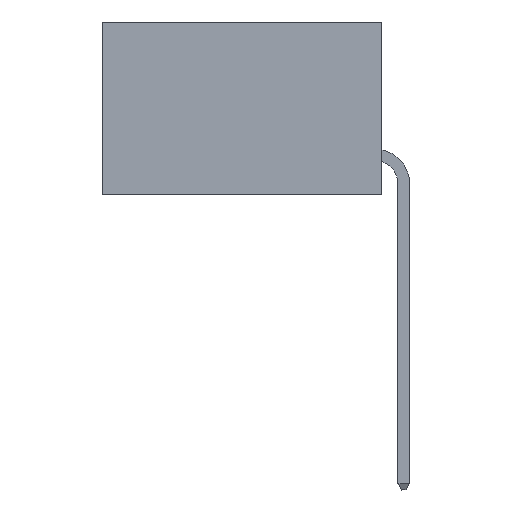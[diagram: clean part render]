
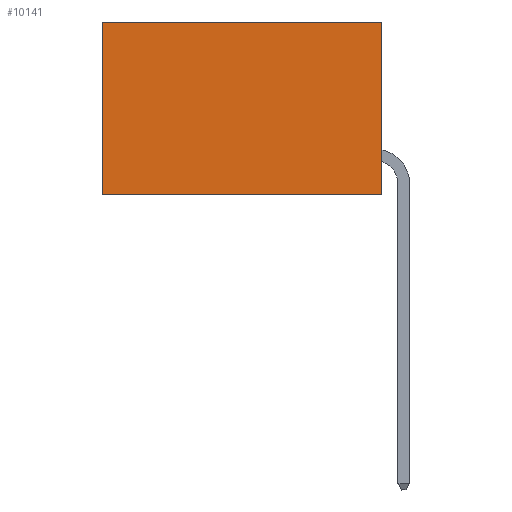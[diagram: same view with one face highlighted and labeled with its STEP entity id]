
A CAD part, left-side view. The second image highlights one B-rep face of the part: STEP entity #10141.
In plain terms, the highlighted planar face has unit normal (-1, 0, 0).
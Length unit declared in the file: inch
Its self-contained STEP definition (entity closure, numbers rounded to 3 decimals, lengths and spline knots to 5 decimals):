
#90 = VERTEX_POINT ( 'NONE', #14069 ) ;
#235 = CARTESIAN_POINT ( 'NONE',  ( 0.2875, 0., 0. ) ) ;
#974 = VERTEX_POINT ( 'NONE', #19655 ) ;
#2861 = VERTEX_POINT ( 'NONE', #24885 ) ;
#3293 = CARTESIAN_POINT ( 'NONE',  ( 0.2875, 0., -0.37 ) ) ;
#5614 = VECTOR ( 'NONE', #13836, 39.37008 ) ;
#5884 = EDGE_CURVE ( 'NONE', #14238, #2861, #18530, .T. ) ;
#6183 = PLANE ( 'NONE',  #18681 ) ;
#7469 = VECTOR ( 'NONE', #16303, 39.37008 ) ;
#7893 = VECTOR ( 'NONE', #18753, 39.37008 ) ;
#8208 = CARTESIAN_POINT ( 'NONE',  ( 0.2875, 0., 0. ) ) ;
#8600 = FACE_OUTER_BOUND ( 'NONE', #19274, .T. ) ;
#8960 = LINE ( 'NONE', #14454, #7469 ) ;
#10034 = ORIENTED_EDGE ( 'NONE', *, *, #5884, .T. ) ;
#10141 = ADVANCED_FACE ( 'NONE', ( #8600 ), #6183, .F. ) ;
#10660 = DIRECTION ( 'NONE',  ( 0., 0., -1. ) ) ;
#10783 = LINE ( 'NONE', #235, #5614 ) ;
#13058 = ORIENTED_EDGE ( 'NONE', *, *, #24590, .F. ) ;
#13836 = DIRECTION ( 'NONE',  ( 0., 0., -1. ) ) ;
#14012 = CARTESIAN_POINT ( 'NONE',  ( 0.2875, 0.6, 0. ) ) ;
#14069 = CARTESIAN_POINT ( 'NONE',  ( 0.2875, 0., 0. ) ) ;
#14238 = VERTEX_POINT ( 'NONE', #14012 ) ;
#14454 = CARTESIAN_POINT ( 'NONE',  ( 0.2875, 0., 0. ) ) ;
#16303 = DIRECTION ( 'NONE',  ( 0., 1., 0. ) ) ;
#16988 = LINE ( 'NONE', #3293, #7893 ) ;
#17162 = EDGE_CURVE ( 'NONE', #90, #14238, #8960, .T. ) ;
#17637 = CARTESIAN_POINT ( 'NONE',  ( 0.2875, 0.6, 0. ) ) ;
#18530 = LINE ( 'NONE', #17637, #20385 ) ;
#18681 = AXIS2_PLACEMENT_3D ( 'NONE', #8208, #19672, #19752 ) ;
#18753 = DIRECTION ( 'NONE',  ( 0., 1., 0. ) ) ;
#19274 = EDGE_LOOP ( 'NONE', ( #10034, #22651, #13058, #23155 ) ) ;
#19655 = CARTESIAN_POINT ( 'NONE',  ( 0.2875, 0., -0.37 ) ) ;
#19672 = DIRECTION ( 'NONE',  ( 1., 0., 0. ) ) ;
#19752 = DIRECTION ( 'NONE',  ( 0., 0., -1. ) ) ;
#20385 = VECTOR ( 'NONE', #10660, 39.37008 ) ;
#20478 = EDGE_CURVE ( 'NONE', #974, #2861, #16988, .T. ) ;
#22651 = ORIENTED_EDGE ( 'NONE', *, *, #20478, .F. ) ;
#23155 = ORIENTED_EDGE ( 'NONE', *, *, #17162, .T. ) ;
#24590 = EDGE_CURVE ( 'NONE', #90, #974, #10783, .T. ) ;
#24885 = CARTESIAN_POINT ( 'NONE',  ( 0.2875, 0.6, -0.37 ) ) ;
